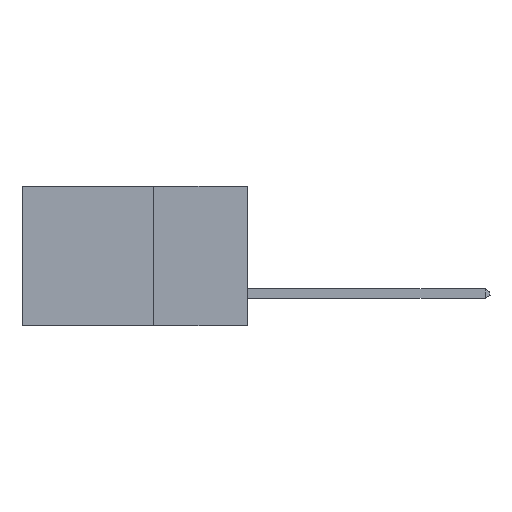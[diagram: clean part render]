
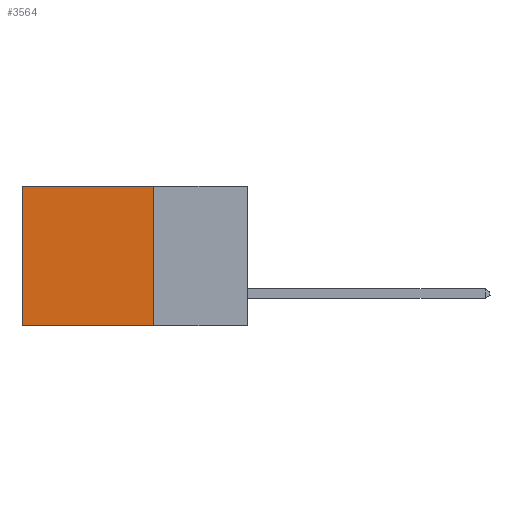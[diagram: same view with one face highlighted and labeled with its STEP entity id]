
A CAD part, left-side view. The second image highlights one B-rep face of the part: STEP entity #3564.
In plain terms, the highlighted planar face has unit normal (-1, 0, 0).
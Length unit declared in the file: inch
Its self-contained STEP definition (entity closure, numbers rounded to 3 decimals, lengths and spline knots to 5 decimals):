
#31 = VECTOR ( 'NONE', #18944, 39.37008 ) ;
#82 = ORIENTED_EDGE ( 'NONE', *, *, #23722, .T. ) ;
#124 = VERTEX_POINT ( 'NONE', #16499 ) ;
#126 = DIRECTION ( 'NONE',  ( 0., 1., 0. ) ) ;
#1361 = AXIS2_PLACEMENT_3D ( 'NONE', #17336, #19724, #26212 ) ;
#2995 = VECTOR ( 'NONE', #6373, 39.37008 ) ;
#3564 = ADVANCED_FACE ( 'NONE', ( #26556 ), #21537, .F. ) ;
#4093 = VECTOR ( 'NONE', #126, 39.37008 ) ;
#6144 = LINE ( 'NONE', #26151, #4093 ) ;
#6373 = DIRECTION ( 'NONE',  ( 0., 1., 0. ) ) ;
#6537 = ORIENTED_EDGE ( 'NONE', *, *, #7444, .F. ) ;
#7444 = EDGE_CURVE ( 'NONE', #17804, #26304, #15355, .T. ) ;
#10442 = EDGE_CURVE ( 'NONE', #17804, #124, #24401, .T. ) ;
#10847 = CARTESIAN_POINT ( 'NONE',  ( 0.298, 0.25, 0. ) ) ;
#12339 = VECTOR ( 'NONE', #26176, 39.37008 ) ;
#14457 = ORIENTED_EDGE ( 'NONE', *, *, #10442, .T. ) ;
#14968 = CARTESIAN_POINT ( 'NONE',  ( 0.298, 0.6, -0.37 ) ) ;
#15210 = CARTESIAN_POINT ( 'NONE',  ( 0.298, 0.25, 0. ) ) ;
#15355 = LINE ( 'NONE', #15210, #12339 ) ;
#15523 = VERTEX_POINT ( 'NONE', #14968 ) ;
#15943 = LINE ( 'NONE', #25531, #31 ) ;
#16023 = EDGE_LOOP ( 'NONE', ( #82, #16585, #6537, #14457 ) ) ;
#16293 = EDGE_CURVE ( 'NONE', #26304, #15523, #6144, .T. ) ;
#16499 = CARTESIAN_POINT ( 'NONE',  ( 0.298, 0.6, 0. ) ) ;
#16585 = ORIENTED_EDGE ( 'NONE', *, *, #16293, .F. ) ;
#17336 = CARTESIAN_POINT ( 'NONE',  ( 0.298, 0.25, 0. ) ) ;
#17804 = VERTEX_POINT ( 'NONE', #26362 ) ;
#18944 = DIRECTION ( 'NONE',  ( 0., 0., -1. ) ) ;
#19724 = DIRECTION ( 'NONE',  ( 1., 0., 0. ) ) ;
#21537 = PLANE ( 'NONE',  #1361 ) ;
#23722 = EDGE_CURVE ( 'NONE', #124, #15523, #15943, .T. ) ;
#24401 = LINE ( 'NONE', #10847, #2995 ) ;
#25531 = CARTESIAN_POINT ( 'NONE',  ( 0.298, 0.6, 0. ) ) ;
#26151 = CARTESIAN_POINT ( 'NONE',  ( 0.298, 0.25, -0.37 ) ) ;
#26176 = DIRECTION ( 'NONE',  ( 0., 0., -1. ) ) ;
#26212 = DIRECTION ( 'NONE',  ( 0., 0., -1. ) ) ;
#26304 = VERTEX_POINT ( 'NONE', #27507 ) ;
#26362 = CARTESIAN_POINT ( 'NONE',  ( 0.298, 0.25, 0. ) ) ;
#26556 = FACE_OUTER_BOUND ( 'NONE', #16023, .T. ) ;
#27507 = CARTESIAN_POINT ( 'NONE',  ( 0.298, 0.25, -0.37 ) ) ;
